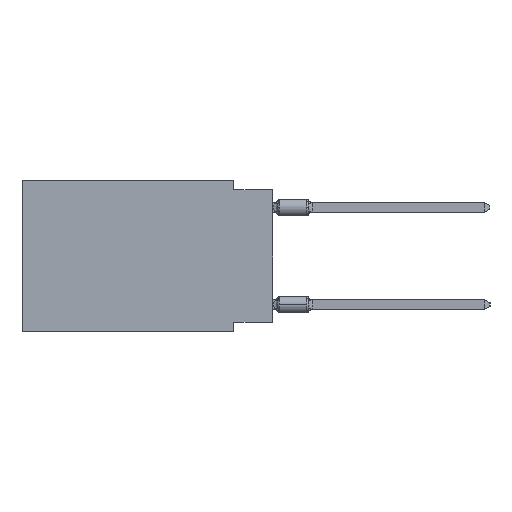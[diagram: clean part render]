
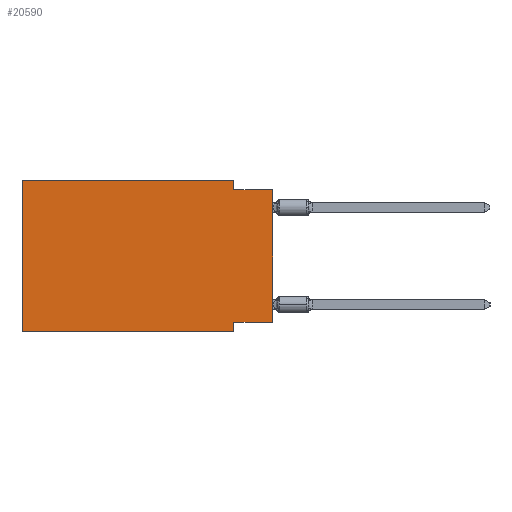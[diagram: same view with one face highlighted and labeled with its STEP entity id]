
A CAD part, left-side view. The second image highlights one B-rep face of the part: STEP entity #20590.
In plain terms, the highlighted planar face has unit normal (-1, 0, 0).
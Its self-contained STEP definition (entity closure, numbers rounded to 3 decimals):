
#175 = CARTESIAN_POINT ( 'NONE',  ( 0., 16.383, 0. ) ) ;
#1775 = CARTESIAN_POINT ( 'NONE',  ( 0., 2.54, 0. ) ) ;
#4243 = ORIENTED_EDGE ( 'NONE', *, *, #9836, .F. ) ;
#4776 = LINE ( 'NONE', #33938, #23827 ) ;
#5265 = VERTEX_POINT ( 'NONE', #21070 ) ;
#5824 = CARTESIAN_POINT ( 'NONE',  ( 0., 16.383, 0. ) ) ;
#6888 = ORIENTED_EDGE ( 'NONE', *, *, #28653, .T. ) ;
#7282 = ORIENTED_EDGE ( 'NONE', *, *, #21706, .F. ) ;
#7474 = CARTESIAN_POINT ( 'NONE',  ( 0., 2.54, -9.271 ) ) ;
#8192 = FACE_OUTER_BOUND ( 'NONE', #32102, .T. ) ;
#8638 = DIRECTION ( 'NONE',  ( 0., 0., 1. ) ) ;
#8979 = VERTEX_POINT ( 'NONE', #26437 ) ;
#9071 = LINE ( 'NONE', #175, #31794 ) ;
#9836 = EDGE_CURVE ( 'NONE', #28305, #5265, #4776, .T. ) ;
#11084 = CARTESIAN_POINT ( 'NONE',  ( 0., 0., -9.271 ) ) ;
#11591 = ORIENTED_EDGE ( 'NONE', *, *, #29831, .F. ) ;
#12509 = DIRECTION ( 'NONE',  ( 0., -1., 0. ) ) ;
#12705 = CARTESIAN_POINT ( 'NONE',  ( 0., 2.54, -9.906 ) ) ;
#13504 = VECTOR ( 'NONE', #8638, 1000. ) ;
#14031 = EDGE_CURVE ( 'NONE', #14351, #28872, #37547, .T. ) ;
#14351 = VERTEX_POINT ( 'NONE', #26907 ) ;
#14432 = CARTESIAN_POINT ( 'NONE',  ( 0., 0., 0. ) ) ;
#14545 = VECTOR ( 'NONE', #12509, 1000. ) ;
#17256 = CARTESIAN_POINT ( 'NONE',  ( 0., 16.383, 0. ) ) ;
#17939 = DIRECTION ( 'NONE',  ( 0., 0., 1. ) ) ;
#18119 = CARTESIAN_POINT ( 'NONE',  ( 0., 16.383, -9.906 ) ) ;
#18843 = CARTESIAN_POINT ( 'NONE',  ( 0., 2.54, 0. ) ) ;
#19968 = DIRECTION ( 'NONE',  ( 0., 0., -1. ) ) ;
#20308 = DIRECTION ( 'NONE',  ( 0., -1., 0. ) ) ;
#20476 = VERTEX_POINT ( 'NONE', #12705 ) ;
#20590 = ADVANCED_FACE ( 'NONE', ( #8192 ), #27750, .F. ) ;
#20855 = EDGE_CURVE ( 'NONE', #36300, #8979, #9071, .T. ) ;
#21070 = CARTESIAN_POINT ( 'NONE',  ( 0., 0., -0.635 ) ) ;
#21329 = VECTOR ( 'NONE', #31179, 1000. ) ;
#21706 = EDGE_CURVE ( 'NONE', #28872, #20476, #24734, .T. ) ;
#21783 = CARTESIAN_POINT ( 'NONE',  ( 0., 2.54, -0.635 ) ) ;
#21982 = VECTOR ( 'NONE', #33618, 1000. ) ;
#22418 = CARTESIAN_POINT ( 'NONE',  ( 0., 2.54, -9.906 ) ) ;
#23827 = VECTOR ( 'NONE', #30854, 1000. ) ;
#24202 = ORIENTED_EDGE ( 'NONE', *, *, #33472, .F. ) ;
#24236 = VERTEX_POINT ( 'NONE', #18843 ) ;
#24487 = LINE ( 'NONE', #18119, #14545 ) ;
#24734 = LINE ( 'NONE', #22418, #21982 ) ;
#25313 = ORIENTED_EDGE ( 'NONE', *, *, #37186, .T. ) ;
#25722 = LINE ( 'NONE', #5824, #28353 ) ;
#26437 = CARTESIAN_POINT ( 'NONE',  ( 0., 16.383, 0. ) ) ;
#26907 = CARTESIAN_POINT ( 'NONE',  ( 0., 0., -9.271 ) ) ;
#27750 = PLANE ( 'NONE',  #32392 ) ;
#27851 = VECTOR ( 'NONE', #34021, 1000. ) ;
#28236 = LINE ( 'NONE', #1775, #27851 ) ;
#28305 = VERTEX_POINT ( 'NONE', #21783 ) ;
#28353 = VECTOR ( 'NONE', #20308, 1000. ) ;
#28653 = EDGE_CURVE ( 'NONE', #36300, #20476, #24487, .T. ) ;
#28872 = VERTEX_POINT ( 'NONE', #7474 ) ;
#29831 = EDGE_CURVE ( 'NONE', #8979, #24236, #25722, .T. ) ;
#30336 = CARTESIAN_POINT ( 'NONE',  ( 0., 16.383, -9.906 ) ) ;
#30854 = DIRECTION ( 'NONE',  ( 0., -1., 0. ) ) ;
#31179 = DIRECTION ( 'NONE',  ( 0., 1., 0. ) ) ;
#31794 = VECTOR ( 'NONE', #17939, 1000. ) ;
#32102 = EDGE_LOOP ( 'NONE', ( #25313, #4243, #24202, #11591, #34412, #6888, #7282, #36913 ) ) ;
#32392 = AXIS2_PLACEMENT_3D ( 'NONE', #17256, #34254, #19968 ) ;
#33472 = EDGE_CURVE ( 'NONE', #24236, #28305, #28236, .T. ) ;
#33618 = DIRECTION ( 'NONE',  ( 0., 0., -1. ) ) ;
#33938 = CARTESIAN_POINT ( 'NONE',  ( 0., 0., -0.635 ) ) ;
#34021 = DIRECTION ( 'NONE',  ( 0., 0., -1. ) ) ;
#34254 = DIRECTION ( 'NONE',  ( 1., 0., 0. ) ) ;
#34412 = ORIENTED_EDGE ( 'NONE', *, *, #20855, .F. ) ;
#34906 = LINE ( 'NONE', #14432, #13504 ) ;
#36300 = VERTEX_POINT ( 'NONE', #30336 ) ;
#36913 = ORIENTED_EDGE ( 'NONE', *, *, #14031, .F. ) ;
#37186 = EDGE_CURVE ( 'NONE', #14351, #5265, #34906, .T. ) ;
#37547 = LINE ( 'NONE', #11084, #21329 ) ;
